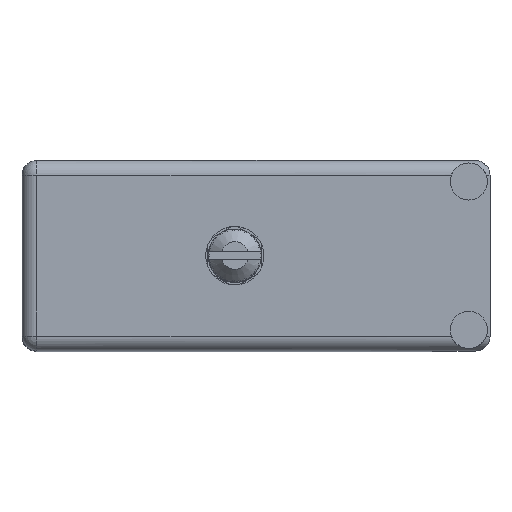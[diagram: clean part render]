
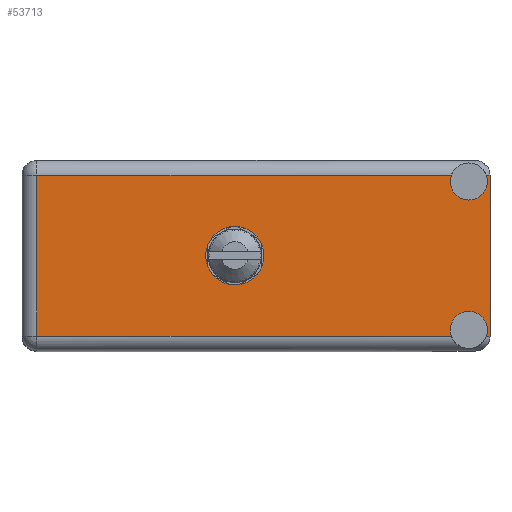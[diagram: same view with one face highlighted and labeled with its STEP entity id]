
A CAD part, top view. The second image highlights one B-rep face of the part: STEP entity #53713.
In plain terms, the highlighted face is planar.
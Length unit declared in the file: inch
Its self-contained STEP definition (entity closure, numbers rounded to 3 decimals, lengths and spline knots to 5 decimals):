
#1419 = DIRECTION ( 'NONE',  ( 0., 0., 1. ) ) ;
#1518 = DIRECTION ( 'NONE',  ( 0., 1., 0. ) ) ;
#1620 = VECTOR ( 'NONE', #96144, 39.37008 ) ;
#2323 = ORIENTED_EDGE ( 'NONE', *, *, #7750, .F. ) ;
#2443 = CARTESIAN_POINT ( 'NONE',  ( 2.108, 1.566, -0.187 ) ) ;
#3686 = LINE ( 'NONE', #19083, #4975 ) ;
#3946 = VERTEX_POINT ( 'NONE', #17970 ) ;
#4146 = EDGE_CURVE ( 'NONE', #15065, #82482, #27402, .T. ) ;
#4157 = ORIENTED_EDGE ( 'NONE', *, *, #94750, .F. ) ;
#4975 = VECTOR ( 'NONE', #75559, 39.37008 ) ;
#5132 = FACE_OUTER_BOUND ( 'NONE', #10422, .T. ) ;
#5662 = AXIS2_PLACEMENT_3D ( 'NONE', #52982, #43788, #100257 ) ;
#6939 = DIRECTION ( 'NONE',  ( 0., 0., 1. ) ) ;
#7750 = EDGE_CURVE ( 'NONE', #101847, #94998, #10694, .T. ) ;
#7823 = ORIENTED_EDGE ( 'NONE', *, *, #60929, .F. ) ;
#7852 = PLANE ( 'NONE',  #61833 ) ;
#9558 = CARTESIAN_POINT ( 'NONE',  ( 1.004, 1.566, -0.4495 ) ) ;
#10158 = CARTESIAN_POINT ( 'NONE',  ( 0.07, 1.566, -0.899 ) ) ;
#10249 = DIRECTION ( 'NONE',  ( 0., 0., 1. ) ) ;
#10422 = EDGE_LOOP ( 'NONE', ( #12640, #2323, #17685, #69277, #101787, #33945, #7823, #4157, #46724, #34224 ) ) ;
#10694 = CIRCLE ( 'NONE', #43452, 0.0875 ) ;
#10718 = EDGE_CURVE ( 'NONE', #91224, #97088, #84923, .T. ) ;
#11243 = CARTESIAN_POINT ( 'NONE',  ( 1.004, 1.566, -0.4495 ) ) ;
#11272 = VECTOR ( 'NONE', #64023, 39.37008 ) ;
#12640 = ORIENTED_EDGE ( 'NONE', *, *, #40644, .T. ) ;
#13979 = CARTESIAN_POINT ( 'NONE',  ( 2.208, 1.566, 0. ) ) ;
#14098 = CARTESIAN_POINT ( 'NONE',  ( 2.19038, 1.566, -0.829 ) ) ;
#15065 = VERTEX_POINT ( 'NONE', #54289 ) ;
#15642 = EDGE_CURVE ( 'NONE', #97088, #91224, #31165, .T. ) ;
#17685 = ORIENTED_EDGE ( 'NONE', *, *, #57105, .F. ) ;
#17970 = CARTESIAN_POINT ( 'NONE',  ( 2.02562, 1.566, -0.829 ) ) ;
#19039 = DIRECTION ( 'NONE',  ( 0., 1., 0. ) ) ;
#19083 = CARTESIAN_POINT ( 'NONE',  ( 0., 1.566, -0.829 ) ) ;
#20799 = ORIENTED_EDGE ( 'NONE', *, *, #15642, .F. ) ;
#23068 = CARTESIAN_POINT ( 'NONE',  ( 2.208, 1.566, -0.07 ) ) ;
#23748 = DIRECTION ( 'NONE',  ( 0., 1., 0. ) ) ;
#24429 = CARTESIAN_POINT ( 'NONE',  ( 2.208, 1.566, -0.07 ) ) ;
#25490 = CIRCLE ( 'NONE', #5662, 0.0875 ) ;
#27402 = LINE ( 'NONE', #13979, #40057 ) ;
#27635 = VERTEX_POINT ( 'NONE', #14098 ) ;
#29991 = LINE ( 'NONE', #10158, #45227 ) ;
#30210 = LINE ( 'NONE', #55938, #11272 ) ;
#30925 = DIRECTION ( 'NONE',  ( 0., 1., 0. ) ) ;
#31165 = CIRCLE ( 'NONE', #100370, 0.1375 ) ;
#31826 = DIRECTION ( 'NONE',  ( 1., 0., 0. ) ) ;
#33945 = ORIENTED_EDGE ( 'NONE', *, *, #98282, .T. ) ;
#34218 = CARTESIAN_POINT ( 'NONE',  ( 2.108, 1.566, -0.0995 ) ) ;
#34224 = ORIENTED_EDGE ( 'NONE', *, *, #87504, .T. ) ;
#34852 = CIRCLE ( 'NONE', #41881, 0.0875 ) ;
#37427 = DIRECTION ( 'NONE',  ( 0., 0., 1. ) ) ;
#40057 = VECTOR ( 'NONE', #95519, 39.37008 ) ;
#40644 = EDGE_CURVE ( 'NONE', #90734, #94998, #75033, .T. ) ;
#41881 = AXIS2_PLACEMENT_3D ( 'NONE', #55013, #30925, #6939 ) ;
#43452 = AXIS2_PLACEMENT_3D ( 'NONE', #92232, #102754, #37427 ) ;
#43788 = DIRECTION ( 'NONE',  ( 0., 1., 0. ) ) ;
#44332 = EDGE_CURVE ( 'NONE', #3946, #57439, #3686, .T. ) ;
#45227 = VECTOR ( 'NONE', #1419, 39.37008 ) ;
#46724 = ORIENTED_EDGE ( 'NONE', *, *, #44332, .T. ) ;
#48432 = LINE ( 'NONE', #103180, #1620 ) ;
#52982 = CARTESIAN_POINT ( 'NONE',  ( 2.108, 1.566, -0.7995 ) ) ;
#53713 = ADVANCED_FACE ( 'NONE', ( #68429, #5132 ), #7852, .T. ) ;
#54289 = CARTESIAN_POINT ( 'NONE',  ( 2.208, 1.566, -0.829 ) ) ;
#55013 = CARTESIAN_POINT ( 'NONE',  ( 2.108, 1.566, -0.7995 ) ) ;
#55938 = CARTESIAN_POINT ( 'NONE',  ( 2.208, 1.566, -0.07 ) ) ;
#56632 = CARTESIAN_POINT ( 'NONE',  ( 2.19038, 1.566, -0.07 ) ) ;
#57105 = EDGE_CURVE ( 'NONE', #92901, #101847, #92838, .T. ) ;
#57439 = VERTEX_POINT ( 'NONE', #82516 ) ;
#60929 = EDGE_CURVE ( 'NONE', #72503, #27635, #25490, .T. ) ;
#61833 = AXIS2_PLACEMENT_3D ( 'NONE', #72476, #23748, #72835 ) ;
#64023 = DIRECTION ( 'NONE',  ( 1., 0., 0. ) ) ;
#66342 = CARTESIAN_POINT ( 'NONE',  ( 2.108, 1.566, -0.712 ) ) ;
#67561 = EDGE_CURVE ( 'NONE', #92901, #82482, #30210, .T. ) ;
#68429 = FACE_BOUND ( 'NONE', #71700, .T. ) ;
#68881 = AXIS2_PLACEMENT_3D ( 'NONE', #11243, #76234, #100219 ) ;
#69277 = ORIENTED_EDGE ( 'NONE', *, *, #67561, .T. ) ;
#71589 = AXIS2_PLACEMENT_3D ( 'NONE', #34218, #19039, #75525 ) ;
#71700 = EDGE_LOOP ( 'NONE', ( #20799, #80657 ) ) ;
#72476 = CARTESIAN_POINT ( 'NONE',  ( 0., 1.566, -0.899 ) ) ;
#72484 = VECTOR ( 'NONE', #31826, 39.37008 ) ;
#72503 = VERTEX_POINT ( 'NONE', #66342 ) ;
#72835 = DIRECTION ( 'NONE',  ( 0., 0., 1. ) ) ;
#73028 = CARTESIAN_POINT ( 'NONE',  ( 1.004, 1.566, -0.312 ) ) ;
#75033 = LINE ( 'NONE', #24429, #72484 ) ;
#75525 = DIRECTION ( 'NONE',  ( 0., 0., 1. ) ) ;
#75559 = DIRECTION ( 'NONE',  ( -1., 0., 0. ) ) ;
#76079 = CARTESIAN_POINT ( 'NONE',  ( 2.02562, 1.566, -0.07 ) ) ;
#76234 = DIRECTION ( 'NONE',  ( 0., 1., 0. ) ) ;
#76444 = CARTESIAN_POINT ( 'NONE',  ( 0.07, 1.566, -0.07 ) ) ;
#78798 = CARTESIAN_POINT ( 'NONE',  ( 1.004, 1.566, -0.587 ) ) ;
#80657 = ORIENTED_EDGE ( 'NONE', *, *, #10718, .F. ) ;
#82482 = VERTEX_POINT ( 'NONE', #23068 ) ;
#82516 = CARTESIAN_POINT ( 'NONE',  ( 0.07, 1.566, -0.829 ) ) ;
#84923 = CIRCLE ( 'NONE', #68881, 0.1375 ) ;
#87504 = EDGE_CURVE ( 'NONE', #57439, #90734, #29991, .T. ) ;
#90734 = VERTEX_POINT ( 'NONE', #76444 ) ;
#91224 = VERTEX_POINT ( 'NONE', #78798 ) ;
#92232 = CARTESIAN_POINT ( 'NONE',  ( 2.108, 1.566, -0.0995 ) ) ;
#92838 = CIRCLE ( 'NONE', #71589, 0.0875 ) ;
#92901 = VERTEX_POINT ( 'NONE', #56632 ) ;
#94750 = EDGE_CURVE ( 'NONE', #3946, #72503, #34852, .T. ) ;
#94998 = VERTEX_POINT ( 'NONE', #76079 ) ;
#95519 = DIRECTION ( 'NONE',  ( 0., 0., 1. ) ) ;
#96144 = DIRECTION ( 'NONE',  ( -1., 0., 0. ) ) ;
#97088 = VERTEX_POINT ( 'NONE', #73028 ) ;
#98282 = EDGE_CURVE ( 'NONE', #15065, #27635, #48432, .T. ) ;
#100219 = DIRECTION ( 'NONE',  ( 0., 0., 1. ) ) ;
#100257 = DIRECTION ( 'NONE',  ( 0., 0., 1. ) ) ;
#100370 = AXIS2_PLACEMENT_3D ( 'NONE', #9558, #1518, #10249 ) ;
#101787 = ORIENTED_EDGE ( 'NONE', *, *, #4146, .F. ) ;
#101847 = VERTEX_POINT ( 'NONE', #2443 ) ;
#102754 = DIRECTION ( 'NONE',  ( 0., 1., 0. ) ) ;
#103180 = CARTESIAN_POINT ( 'NONE',  ( 0., 1.566, -0.829 ) ) ;
